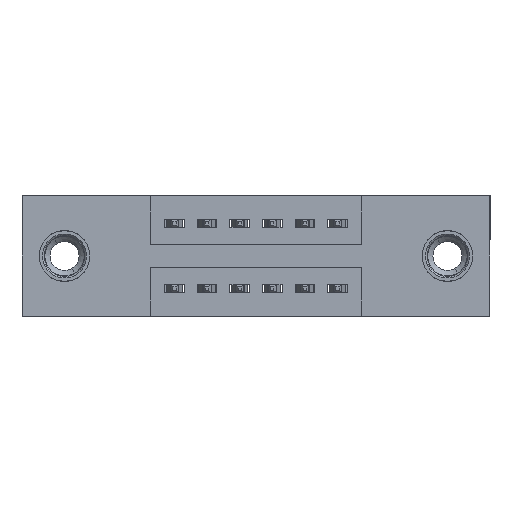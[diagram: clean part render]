
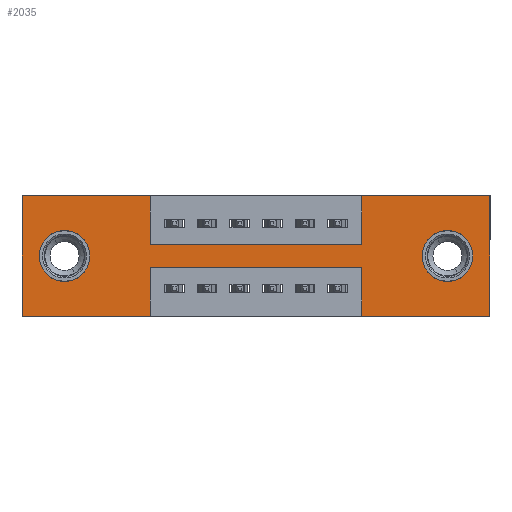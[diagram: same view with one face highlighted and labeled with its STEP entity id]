
A CAD part, front view. The second image highlights one B-rep face of the part: STEP entity #2035.
In plain terms, the highlighted planar face has unit normal (0, -1, 0).
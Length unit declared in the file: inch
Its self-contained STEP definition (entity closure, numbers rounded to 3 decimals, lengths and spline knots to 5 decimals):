
#14 = LINE ( 'NONE', #9853, #8486 ) ;
#137 = CARTESIAN_POINT ( 'NONE',  ( 0.3925, 0., -0.22 ) ) ;
#453 = CARTESIAN_POINT ( 'NONE',  ( 1.435, 0., 0. ) ) ;
#465 = EDGE_CURVE ( 'NONE', #3998, #6371, #7043, .T. ) ;
#552 = CARTESIAN_POINT ( 'NONE',  ( 0.13, 0., -0.107 ) ) ;
#756 = ORIENTED_EDGE ( 'NONE', *, *, #1414, .T. ) ;
#815 = EDGE_CURVE ( 'NONE', #3979, #6585, #12070, .T. ) ;
#879 = EDGE_LOOP ( 'NONE', ( #3042, #4907, #12342, #14286, #7978, #2398, #10056, #13436, #9574, #3647, #7193, #2235 ) ) ;
#992 = CARTESIAN_POINT ( 'NONE',  ( 0., 0., -0.37 ) ) ;
#1080 = CARTESIAN_POINT ( 'NONE',  ( 0., 0., 0. ) ) ;
#1285 = LINE ( 'NONE', #137, #5441 ) ;
#1414 = EDGE_CURVE ( 'NONE', #5386, #3338, #9755, .T. ) ;
#1721 = LINE ( 'NONE', #11267, #8120 ) ;
#1906 = DIRECTION ( 'NONE',  ( 0., 0., -1. ) ) ;
#2035 = ADVANCED_FACE ( 'NONE', ( #2842, #7633, #13583 ), #5737, .T. ) ;
#2235 = ORIENTED_EDGE ( 'NONE', *, *, #11908, .F. ) ;
#2293 = EDGE_LOOP ( 'NONE', ( #12101, #8366 ) ) ;
#2398 = ORIENTED_EDGE ( 'NONE', *, *, #9238, .F. ) ;
#2490 = CARTESIAN_POINT ( 'NONE',  ( 0., 0., -0.37 ) ) ;
#2621 = EDGE_LOOP ( 'NONE', ( #9580, #756 ) ) ;
#2842 = FACE_BOUND ( 'NONE', #2293, .T. ) ;
#3040 = VERTEX_POINT ( 'NONE', #1080 ) ;
#3042 = ORIENTED_EDGE ( 'NONE', *, *, #12370, .F. ) ;
#3108 = DIRECTION ( 'NONE',  ( 1., 0., 0. ) ) ;
#3222 = EDGE_CURVE ( 'NONE', #5412, #3979, #10499, .T. ) ;
#3330 = CARTESIAN_POINT ( 'NONE',  ( 1.305, 0., -0.185 ) ) ;
#3338 = VERTEX_POINT ( 'NONE', #552 ) ;
#3466 = VERTEX_POINT ( 'NONE', #8567 ) ;
#3647 = ORIENTED_EDGE ( 'NONE', *, *, #11638, .F. ) ;
#3818 = LINE ( 'NONE', #992, #7950 ) ;
#3895 = VECTOR ( 'NONE', #3108, 39.37008 ) ;
#3979 = VERTEX_POINT ( 'NONE', #9565 ) ;
#3998 = VERTEX_POINT ( 'NONE', #4070 ) ;
#4013 = DIRECTION ( 'NONE',  ( 0., 1., 0. ) ) ;
#4070 = CARTESIAN_POINT ( 'NONE',  ( 0.3925, 0., -0.15 ) ) ;
#4079 = DIRECTION ( 'NONE',  ( 0., 0., -1. ) ) ;
#4084 = CARTESIAN_POINT ( 'NONE',  ( 0., 0., 0. ) ) ;
#4141 = VECTOR ( 'NONE', #14342, 39.37008 ) ;
#4709 = DIRECTION ( 'NONE',  ( 0., 0., -1. ) ) ;
#4734 = VERTEX_POINT ( 'NONE', #11470 ) ;
#4797 = CARTESIAN_POINT ( 'NONE',  ( 1.0425, 0., -0.15 ) ) ;
#4907 = ORIENTED_EDGE ( 'NONE', *, *, #8804, .F. ) ;
#5213 = EDGE_CURVE ( 'NONE', #9485, #3998, #1721, .T. ) ;
#5294 = EDGE_CURVE ( 'NONE', #12944, #3040, #7944, .T. ) ;
#5386 = VERTEX_POINT ( 'NONE', #11523 ) ;
#5389 = VERTEX_POINT ( 'NONE', #8148 ) ;
#5412 = VERTEX_POINT ( 'NONE', #9359 ) ;
#5441 = VECTOR ( 'NONE', #5733, 39.37008 ) ;
#5447 = AXIS2_PLACEMENT_3D ( 'NONE', #3330, #10999, #13242 ) ;
#5681 = DIRECTION ( 'NONE',  ( 0., 0., 1. ) ) ;
#5733 = DIRECTION ( 'NONE',  ( -1., 0., 0. ) ) ;
#5737 = PLANE ( 'NONE',  #13326 ) ;
#5791 = CARTESIAN_POINT ( 'NONE',  ( 0.13, 0., -0.185 ) ) ;
#6171 = VECTOR ( 'NONE', #12108, 39.37008 ) ;
#6190 = EDGE_CURVE ( 'NONE', #6585, #3466, #13676, .T. ) ;
#6194 = CARTESIAN_POINT ( 'NONE',  ( 0.13, 0., -0.185 ) ) ;
#6371 = VERTEX_POINT ( 'NONE', #4797 ) ;
#6543 = EDGE_CURVE ( 'NONE', #5389, #10705, #12817, .T. ) ;
#6585 = VERTEX_POINT ( 'NONE', #12236 ) ;
#6878 = DIRECTION ( 'NONE',  ( 0., 1., 0. ) ) ;
#6922 = DIRECTION ( 'NONE',  ( 0., 0., -1. ) ) ;
#6977 = DIRECTION ( 'NONE',  ( 0., 0., 1. ) ) ;
#7026 = EDGE_CURVE ( 'NONE', #6371, #4734, #10157, .T. ) ;
#7043 = LINE ( 'NONE', #10955, #4141 ) ;
#7193 = ORIENTED_EDGE ( 'NONE', *, *, #5294, .F. ) ;
#7633 = FACE_BOUND ( 'NONE', #2621, .T. ) ;
#7813 = CARTESIAN_POINT ( 'NONE',  ( 0.3925, 0., -0.22 ) ) ;
#7840 = LINE ( 'NONE', #4084, #3895 ) ;
#7878 = VERTEX_POINT ( 'NONE', #7813 ) ;
#7944 = LINE ( 'NONE', #12457, #14215 ) ;
#7950 = VECTOR ( 'NONE', #10932, 39.37008 ) ;
#7978 = ORIENTED_EDGE ( 'NONE', *, *, #3222, .F. ) ;
#8107 = DIRECTION ( 'NONE',  ( 0., -1., 0. ) ) ;
#8120 = VECTOR ( 'NONE', #4709, 39.37008 ) ;
#8148 = CARTESIAN_POINT ( 'NONE',  ( 1.305, 0., -0.263 ) ) ;
#8366 = ORIENTED_EDGE ( 'NONE', *, *, #6543, .T. ) ;
#8427 = DIRECTION ( 'NONE',  ( 1., 0., 0. ) ) ;
#8486 = VECTOR ( 'NONE', #8427, 39.37008 ) ;
#8537 = VECTOR ( 'NONE', #12607, 39.37008 ) ;
#8559 = VECTOR ( 'NONE', #12484, 39.37008 ) ;
#8567 = CARTESIAN_POINT ( 'NONE',  ( 1.0425, 0., -0.22 ) ) ;
#8804 = EDGE_CURVE ( 'NONE', #3466, #7878, #1285, .T. ) ;
#8915 = CARTESIAN_POINT ( 'NONE',  ( 1.305, 0., -0.107 ) ) ;
#9238 = EDGE_CURVE ( 'NONE', #4734, #5412, #7840, .T. ) ;
#9359 = CARTESIAN_POINT ( 'NONE',  ( 1.435, 0., 0. ) ) ;
#9485 = VERTEX_POINT ( 'NONE', #10243 ) ;
#9565 = CARTESIAN_POINT ( 'NONE',  ( 1.435, 0., -0.37 ) ) ;
#9574 = ORIENTED_EDGE ( 'NONE', *, *, #5213, .F. ) ;
#9580 = ORIENTED_EDGE ( 'NONE', *, *, #10779, .T. ) ;
#9755 = CIRCLE ( 'NONE', #12891, 0.078 ) ;
#9853 = CARTESIAN_POINT ( 'NONE',  ( 0., 0., 0. ) ) ;
#10056 = ORIENTED_EDGE ( 'NONE', *, *, #7026, .F. ) ;
#10157 = LINE ( 'NONE', #11179, #10517 ) ;
#10243 = CARTESIAN_POINT ( 'NONE',  ( 0.3925, 0., 0. ) ) ;
#10323 = AXIS2_PLACEMENT_3D ( 'NONE', #5791, #6878, #6977 ) ;
#10499 = LINE ( 'NONE', #453, #8537 ) ;
#10517 = VECTOR ( 'NONE', #13810, 39.37008 ) ;
#10657 = CARTESIAN_POINT ( 'NONE',  ( 1.305, 0., -0.185 ) ) ;
#10705 = VERTEX_POINT ( 'NONE', #8915 ) ;
#10779 = EDGE_CURVE ( 'NONE', #3338, #5386, #11499, .T. ) ;
#10932 = DIRECTION ( 'NONE',  ( -1., 0., 0. ) ) ;
#10955 = CARTESIAN_POINT ( 'NONE',  ( 0.3925, 0., -0.15 ) ) ;
#10999 = DIRECTION ( 'NONE',  ( 0., 1., 0. ) ) ;
#11179 = CARTESIAN_POINT ( 'NONE',  ( 1.0425, 0., 0. ) ) ;
#11267 = CARTESIAN_POINT ( 'NONE',  ( 0.3925, 0., 0. ) ) ;
#11470 = CARTESIAN_POINT ( 'NONE',  ( 1.0425, 0., 0. ) ) ;
#11499 = CIRCLE ( 'NONE', #10323, 0.078 ) ;
#11523 = CARTESIAN_POINT ( 'NONE',  ( 0.13, 0., -0.263 ) ) ;
#11638 = EDGE_CURVE ( 'NONE', #3040, #9485, #14, .T. ) ;
#11755 = VERTEX_POINT ( 'NONE', #13973 ) ;
#11846 = CARTESIAN_POINT ( 'NONE',  ( 0.3925, 0., -0.37 ) ) ;
#11906 = CIRCLE ( 'NONE', #14122, 0.078 ) ;
#11908 = EDGE_CURVE ( 'NONE', #11755, #12944, #3818, .T. ) ;
#12070 = LINE ( 'NONE', #13722, #8559 ) ;
#12101 = ORIENTED_EDGE ( 'NONE', *, *, #12553, .T. ) ;
#12108 = DIRECTION ( 'NONE',  ( 0., 0., 1. ) ) ;
#12236 = CARTESIAN_POINT ( 'NONE',  ( 1.0425, 0., -0.37 ) ) ;
#12246 = VECTOR ( 'NONE', #4079, 39.37008 ) ;
#12342 = ORIENTED_EDGE ( 'NONE', *, *, #6190, .F. ) ;
#12370 = EDGE_CURVE ( 'NONE', #7878, #11755, #12619, .T. ) ;
#12457 = CARTESIAN_POINT ( 'NONE',  ( 0., 0., 0. ) ) ;
#12484 = DIRECTION ( 'NONE',  ( -1., 0., 0. ) ) ;
#12553 = EDGE_CURVE ( 'NONE', #10705, #5389, #11906, .T. ) ;
#12607 = DIRECTION ( 'NONE',  ( 0., 0., -1. ) ) ;
#12619 = LINE ( 'NONE', #11846, #12246 ) ;
#12814 = DIRECTION ( 'NONE',  ( 0., 1., 0. ) ) ;
#12817 = CIRCLE ( 'NONE', #5447, 0.078 ) ;
#12866 = DIRECTION ( 'NONE',  ( 0., 0., 1. ) ) ;
#12891 = AXIS2_PLACEMENT_3D ( 'NONE', #6194, #12814, #12866 ) ;
#12944 = VERTEX_POINT ( 'NONE', #2490 ) ;
#13242 = DIRECTION ( 'NONE',  ( 0., 0., -1. ) ) ;
#13326 = AXIS2_PLACEMENT_3D ( 'NONE', #13615, #8107, #6922 ) ;
#13436 = ORIENTED_EDGE ( 'NONE', *, *, #465, .F. ) ;
#13583 = FACE_OUTER_BOUND ( 'NONE', #879, .T. ) ;
#13615 = CARTESIAN_POINT ( 'NONE',  ( 0., 0., -0.37 ) ) ;
#13676 = LINE ( 'NONE', #14275, #6171 ) ;
#13722 = CARTESIAN_POINT ( 'NONE',  ( 0., 0., -0.37 ) ) ;
#13810 = DIRECTION ( 'NONE',  ( 0., 0., 1. ) ) ;
#13973 = CARTESIAN_POINT ( 'NONE',  ( 0.3925, 0., -0.37 ) ) ;
#14122 = AXIS2_PLACEMENT_3D ( 'NONE', #10657, #4013, #1906 ) ;
#14215 = VECTOR ( 'NONE', #5681, 39.37008 ) ;
#14275 = CARTESIAN_POINT ( 'NONE',  ( 1.0425, 0., -0.37 ) ) ;
#14286 = ORIENTED_EDGE ( 'NONE', *, *, #815, .F. ) ;
#14342 = DIRECTION ( 'NONE',  ( 1., 0., 0. ) ) ;
